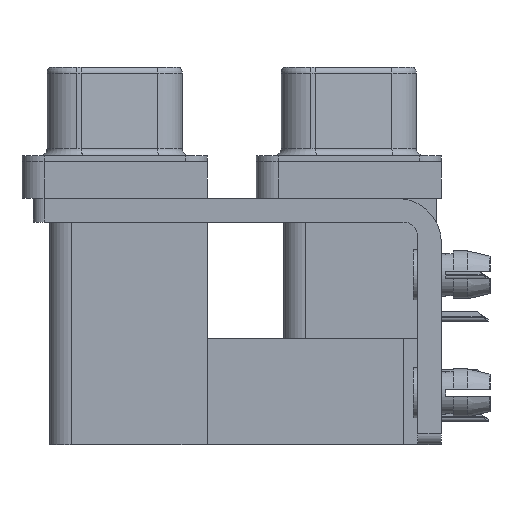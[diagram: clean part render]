
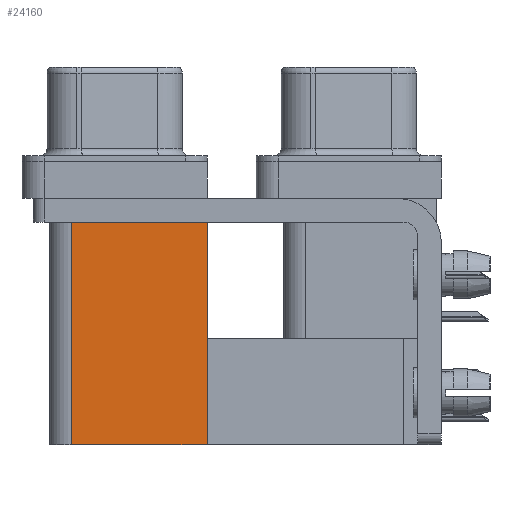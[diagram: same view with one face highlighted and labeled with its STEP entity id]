
A CAD part, left-side view. The second image highlights one B-rep face of the part: STEP entity #24160.
In plain terms, the highlighted planar face has unit normal (-1, 0, 0).
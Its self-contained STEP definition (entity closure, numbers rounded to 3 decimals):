
#111 = CARTESIAN_POINT ( 'NONE',  ( 3.7, 9.6, -19.2 ) ) ;
#516 = ORIENTED_EDGE ( 'NONE', *, *, #26850, .T. ) ;
#1118 = CARTESIAN_POINT ( 'NONE',  ( 3.7, 18.8, -2.5 ) ) ;
#1329 = EDGE_LOOP ( 'NONE', ( #19237, #38276, #41113, #516 ) ) ;
#1372 = DIRECTION ( 'NONE',  ( 0., 1., 0. ) ) ;
#1626 = VECTOR ( 'NONE', #1372, 1000. ) ;
#2517 = DIRECTION ( 'NONE',  ( 0., 1., 0. ) ) ;
#5452 = CARTESIAN_POINT ( 'NONE',  ( 3.7, 9.6, -19.2 ) ) ;
#5569 = EDGE_CURVE ( 'NONE', #34313, #30346, #34186, .T. ) ;
#6297 = PLANE ( 'NONE',  #9638 ) ;
#7788 = VECTOR ( 'NONE', #11391, 1000. ) ;
#9638 = AXIS2_PLACEMENT_3D ( 'NONE', #22253, #16064, #29060 ) ;
#11391 = DIRECTION ( 'NONE',  ( 0., 0., 1. ) ) ;
#12023 = LINE ( 'NONE', #5452, #7788 ) ;
#14386 = VECTOR ( 'NONE', #39009, 1000. ) ;
#16064 = DIRECTION ( 'NONE',  ( 1., 0., 0. ) ) ;
#19237 = ORIENTED_EDGE ( 'NONE', *, *, #5569, .T. ) ;
#19798 = LINE ( 'NONE', #32806, #14386 ) ;
#20310 = CARTESIAN_POINT ( 'NONE',  ( 3.7, 9.6, -2.5 ) ) ;
#20481 = VECTOR ( 'NONE', #2517, 1000. ) ;
#22065 = LINE ( 'NONE', #41280, #20481 ) ;
#22253 = CARTESIAN_POINT ( 'NONE',  ( 3.7, 9.6, -19.2 ) ) ;
#24160 = ADVANCED_FACE ( 'NONE', ( #25438 ), #6297, .F. ) ;
#24426 = CARTESIAN_POINT ( 'NONE',  ( 3.7, 9.6, -2.5 ) ) ;
#25438 = FACE_OUTER_BOUND ( 'NONE', #1329, .T. ) ;
#26850 = EDGE_CURVE ( 'NONE', #27884, #34313, #12023, .T. ) ;
#27884 = VERTEX_POINT ( 'NONE', #111 ) ;
#29060 = DIRECTION ( 'NONE',  ( 0., 0., -1. ) ) ;
#30346 = VERTEX_POINT ( 'NONE', #1118 ) ;
#32806 = CARTESIAN_POINT ( 'NONE',  ( 3.7, 18.8, -19.2 ) ) ;
#34031 = VERTEX_POINT ( 'NONE', #36016 ) ;
#34186 = LINE ( 'NONE', #20310, #1626 ) ;
#34313 = VERTEX_POINT ( 'NONE', #24426 ) ;
#34472 = EDGE_CURVE ( 'NONE', #27884, #34031, #22065, .T. ) ;
#35799 = EDGE_CURVE ( 'NONE', #34031, #30346, #19798, .T. ) ;
#36016 = CARTESIAN_POINT ( 'NONE',  ( 3.7, 18.8, -19.2 ) ) ;
#38276 = ORIENTED_EDGE ( 'NONE', *, *, #35799, .F. ) ;
#39009 = DIRECTION ( 'NONE',  ( 0., 0., 1. ) ) ;
#41113 = ORIENTED_EDGE ( 'NONE', *, *, #34472, .F. ) ;
#41280 = CARTESIAN_POINT ( 'NONE',  ( 3.7, 9.6, -19.2 ) ) ;
